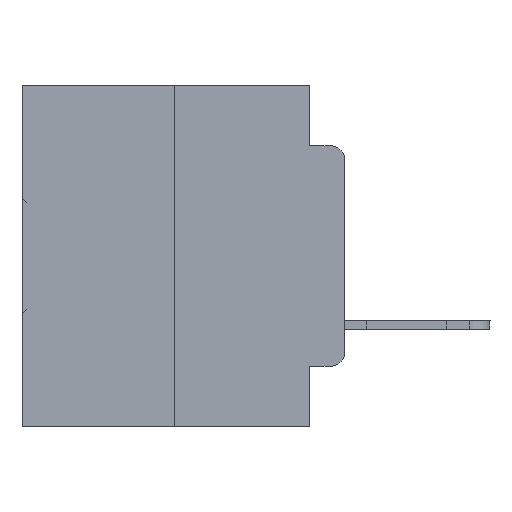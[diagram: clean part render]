
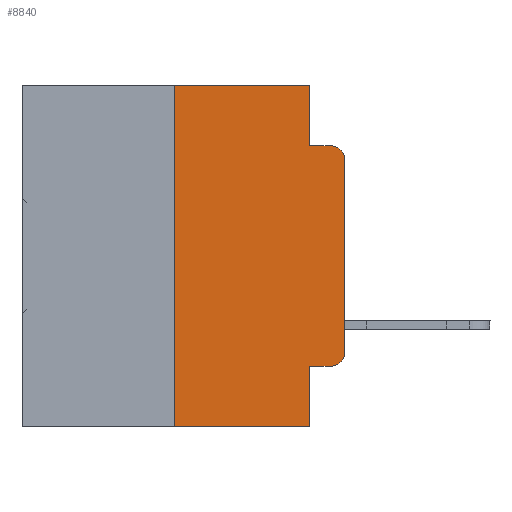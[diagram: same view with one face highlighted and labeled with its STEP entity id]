
A CAD part, left-side view. The second image highlights one B-rep face of the part: STEP entity #8840.
In plain terms, the highlighted planar face has unit normal (-1, 0, 0).
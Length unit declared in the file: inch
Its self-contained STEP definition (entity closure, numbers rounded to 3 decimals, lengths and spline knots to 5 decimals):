
#1528 = DIRECTION ( 'NONE',  ( 0., -1., 0. ) ) ;
#1946 = DIRECTION ( 'NONE',  ( 0., 0., -1. ) ) ;
#2393 = DIRECTION ( 'NONE',  ( 0., 0., -1. ) ) ;
#2432 = CARTESIAN_POINT ( 'NONE',  ( 0., 0.25, 0. ) ) ;
#2592 = ORIENTED_EDGE ( 'NONE', *, *, #8692, .T. ) ;
#2690 = DIRECTION ( 'NONE',  ( 0., -1., 0. ) ) ;
#2763 = DIRECTION ( 'NONE',  ( 0., 0., 1. ) ) ;
#4266 = AXIS2_PLACEMENT_3D ( 'NONE', #8188, #16733, #24339 ) ;
#4681 = ORIENTED_EDGE ( 'NONE', *, *, #21913, .F. ) ;
#4694 = AXIS2_PLACEMENT_3D ( 'NONE', #23912, #18391, #10025 ) ;
#4937 = VERTEX_POINT ( 'NONE', #11831 ) ;
#5646 = CARTESIAN_POINT ( 'NONE',  ( 0., 0.051, 0. ) ) ;
#6201 = FACE_OUTER_BOUND ( 'NONE', #12659, .T. ) ;
#6718 = CARTESIAN_POINT ( 'NONE',  ( 0., 0.25, -0.5 ) ) ;
#6759 = CARTESIAN_POINT ( 'NONE',  ( 0., 0.473, 0. ) ) ;
#7372 = ORIENTED_EDGE ( 'NONE', *, *, #25666, .T. ) ;
#7406 = LINE ( 'NONE', #27800, #14160 ) ;
#7901 = VECTOR ( 'NONE', #12112, 39.37008 ) ;
#8174 = CARTESIAN_POINT ( 'NONE',  ( 0., 0., -0.1085 ) ) ;
#8188 = CARTESIAN_POINT ( 'NONE',  ( 0., 0.473, 0. ) ) ;
#8515 = PLANE ( 'NONE',  #4266 ) ;
#8692 = EDGE_CURVE ( 'NONE', #17546, #21604, #21962, .T. ) ;
#8728 = CARTESIAN_POINT ( 'NONE',  ( 0., 0.051, -0.5 ) ) ;
#8840 = ADVANCED_FACE ( 'NONE', ( #6201 ), #8515, .F. ) ;
#10025 = DIRECTION ( 'NONE',  ( 0., 0., -1. ) ) ;
#10707 = ORIENTED_EDGE ( 'NONE', *, *, #34742, .T. ) ;
#11125 = VERTEX_POINT ( 'NONE', #26916 ) ;
#11831 = CARTESIAN_POINT ( 'NONE',  ( 0., 0.051, -0.4115 ) ) ;
#12005 = VECTOR ( 'NONE', #1528, 39.37008 ) ;
#12112 = DIRECTION ( 'NONE',  ( 0., -1., 0. ) ) ;
#12659 = EDGE_LOOP ( 'NONE', ( #10707, #28603, #14489, #4681, #18915, #18358, #2592, #30562, #7372, #33989 ) ) ;
#13036 = VECTOR ( 'NONE', #34427, 39.37008 ) ;
#13242 = DIRECTION ( 'NONE',  ( -1., 0., 0. ) ) ;
#13278 = CARTESIAN_POINT ( 'NONE',  ( 0., 0.051, 0. ) ) ;
#13502 = EDGE_CURVE ( 'NONE', #34278, #31766, #28983, .T. ) ;
#14160 = VECTOR ( 'NONE', #17062, 39.37008 ) ;
#14489 = ORIENTED_EDGE ( 'NONE', *, *, #13502, .F. ) ;
#14933 = EDGE_CURVE ( 'NONE', #4937, #21604, #16590, .T. ) ;
#15125 = LINE ( 'NONE', #6759, #7901 ) ;
#16061 = CARTESIAN_POINT ( 'NONE',  ( 0., 0.473, -0.5 ) ) ;
#16180 = CIRCLE ( 'NONE', #21385, 0.02 ) ;
#16217 = VERTEX_POINT ( 'NONE', #29123 ) ;
#16590 = LINE ( 'NONE', #24939, #20022 ) ;
#16723 = VERTEX_POINT ( 'NONE', #8174 ) ;
#16733 = DIRECTION ( 'NONE',  ( 1., 0., 0. ) ) ;
#17062 = DIRECTION ( 'NONE',  ( 0., -1., 0. ) ) ;
#17546 = VERTEX_POINT ( 'NONE', #6718 ) ;
#17863 = CARTESIAN_POINT ( 'NONE',  ( 0., 0.051, -0.0885 ) ) ;
#18358 = ORIENTED_EDGE ( 'NONE', *, *, #26184, .F. ) ;
#18391 = DIRECTION ( 'NONE',  ( -1., 0., 0. ) ) ;
#18915 = ORIENTED_EDGE ( 'NONE', *, *, #19992, .F. ) ;
#19290 = CARTESIAN_POINT ( 'NONE',  ( 0., 0.051, -0.0885 ) ) ;
#19992 = EDGE_CURVE ( 'NONE', #16217, #28498, #15125, .T. ) ;
#20022 = VECTOR ( 'NONE', #22479, 39.37008 ) ;
#20047 = CARTESIAN_POINT ( 'NONE',  ( 0., 0.02, -0.0885 ) ) ;
#21275 = CIRCLE ( 'NONE', #4694, 0.02 ) ;
#21385 = AXIS2_PLACEMENT_3D ( 'NONE', #26473, #13242, #2393 ) ;
#21604 = VERTEX_POINT ( 'NONE', #8728 ) ;
#21801 = VECTOR ( 'NONE', #2763, 39.37008 ) ;
#21913 = EDGE_CURVE ( 'NONE', #28498, #34278, #27634, .T. ) ;
#21962 = LINE ( 'NONE', #16061, #30782 ) ;
#22479 = DIRECTION ( 'NONE',  ( 0., 0., -1. ) ) ;
#23912 = CARTESIAN_POINT ( 'NONE',  ( 0., 0.02, -0.1085 ) ) ;
#24339 = DIRECTION ( 'NONE',  ( 0., 0., -1. ) ) ;
#24939 = CARTESIAN_POINT ( 'NONE',  ( 0., 0.051, 0. ) ) ;
#25120 = LINE ( 'NONE', #2432, #21801 ) ;
#25666 = EDGE_CURVE ( 'NONE', #4937, #30867, #7406, .T. ) ;
#26096 = CARTESIAN_POINT ( 'NONE',  ( 0., 0., 0. ) ) ;
#26184 = EDGE_CURVE ( 'NONE', #17546, #16217, #25120, .T. ) ;
#26473 = CARTESIAN_POINT ( 'NONE',  ( 0., 0.02, -0.3915 ) ) ;
#26916 = CARTESIAN_POINT ( 'NONE',  ( 0., 0., -0.3915 ) ) ;
#27634 = LINE ( 'NONE', #13278, #34388 ) ;
#27637 = EDGE_CURVE ( 'NONE', #16723, #31766, #21275, .T. ) ;
#27800 = CARTESIAN_POINT ( 'NONE',  ( 0., 0.051, -0.4115 ) ) ;
#28498 = VERTEX_POINT ( 'NONE', #5646 ) ;
#28603 = ORIENTED_EDGE ( 'NONE', *, *, #27637, .T. ) ;
#28983 = LINE ( 'NONE', #17863, #12005 ) ;
#29123 = CARTESIAN_POINT ( 'NONE',  ( 0., 0.25, 0. ) ) ;
#29814 = CARTESIAN_POINT ( 'NONE',  ( 0., 0.02, -0.4115 ) ) ;
#30562 = ORIENTED_EDGE ( 'NONE', *, *, #14933, .F. ) ;
#30782 = VECTOR ( 'NONE', #2690, 39.37008 ) ;
#30867 = VERTEX_POINT ( 'NONE', #29814 ) ;
#31766 = VERTEX_POINT ( 'NONE', #20047 ) ;
#33693 = EDGE_CURVE ( 'NONE', #30867, #11125, #16180, .T. ) ;
#33989 = ORIENTED_EDGE ( 'NONE', *, *, #33693, .T. ) ;
#34278 = VERTEX_POINT ( 'NONE', #19290 ) ;
#34388 = VECTOR ( 'NONE', #1946, 39.37008 ) ;
#34427 = DIRECTION ( 'NONE',  ( 0., 0., 1. ) ) ;
#34560 = LINE ( 'NONE', #26096, #13036 ) ;
#34742 = EDGE_CURVE ( 'NONE', #11125, #16723, #34560, .T. ) ;
